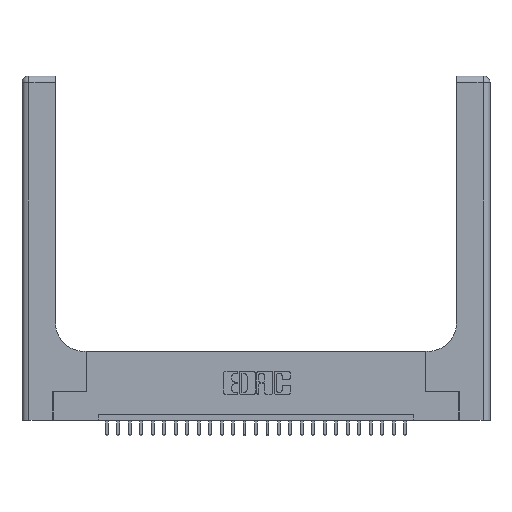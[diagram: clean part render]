
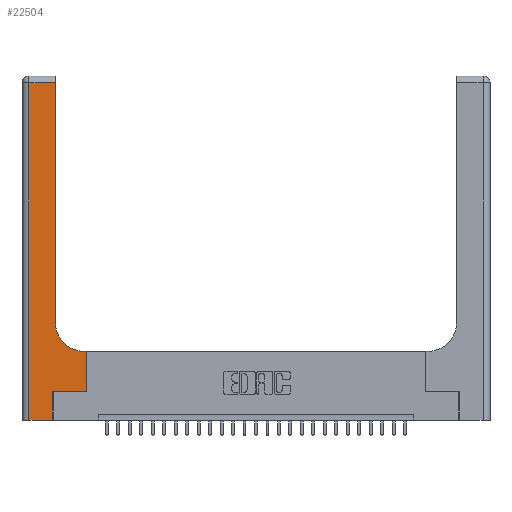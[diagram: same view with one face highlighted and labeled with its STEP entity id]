
A CAD part, top view. The second image highlights one B-rep face of the part: STEP entity #22504.
In plain terms, the highlighted planar face has unit normal (0, 0, 1).
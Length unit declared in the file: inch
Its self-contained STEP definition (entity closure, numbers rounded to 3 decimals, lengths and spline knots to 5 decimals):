
#38 = VECTOR ( 'NONE', #24473, 39.37008 ) ;
#430 = DIRECTION ( 'NONE',  ( -1., 0., 0. ) ) ;
#1986 = LINE ( 'NONE', #11225, #23203 ) ;
#2425 = CIRCLE ( 'NONE', #13487, 0.25 ) ;
#2808 = EDGE_CURVE ( 'NONE', #12086, #2847, #2425, .T. ) ;
#2847 = VERTEX_POINT ( 'NONE', #17193 ) ;
#3329 = VECTOR ( 'NONE', #17822, 39.37008 ) ;
#3611 = VERTEX_POINT ( 'NONE', #10366 ) ;
#3762 = ORIENTED_EDGE ( 'NONE', *, *, #16339, .T. ) ;
#4266 = ORIENTED_EDGE ( 'NONE', *, *, #25864, .T. ) ;
#4330 = CARTESIAN_POINT ( 'NONE',  ( 0.269, 0., 0.37 ) ) ;
#4555 = LINE ( 'NONE', #6784, #12500 ) ;
#5324 = CARTESIAN_POINT ( 'NONE',  ( 0.5585, 0.25, 0.37 ) ) ;
#5474 = CARTESIAN_POINT ( 'NONE',  ( 0., 0., 0.37 ) ) ;
#5897 = ORIENTED_EDGE ( 'NONE', *, *, #21967, .T. ) ;
#6282 = DIRECTION ( 'NONE',  ( 1., 0., 0. ) ) ;
#6784 = CARTESIAN_POINT ( 'NONE',  ( 0.2915, 3., 0.37 ) ) ;
#9397 = ORIENTED_EDGE ( 'NONE', *, *, #18760, .T. ) ;
#9572 = EDGE_LOOP ( 'NONE', ( #24505, #5897, #26247, #18414, #4266, #3762, #9597, #9397, #11626 ) ) ;
#9597 = ORIENTED_EDGE ( 'NONE', *, *, #9991, .T. ) ;
#9695 = CARTESIAN_POINT ( 'NONE',  ( 0.06, 3., 0.37 ) ) ;
#9987 = LINE ( 'NONE', #9695, #14293 ) ;
#9991 = EDGE_CURVE ( 'NONE', #10558, #22808, #16920, .T. ) ;
#10335 = DIRECTION ( 'NONE',  ( 0., 0., -1. ) ) ;
#10366 = CARTESIAN_POINT ( 'NONE',  ( 0.269, 0., 0.37 ) ) ;
#10558 = VERTEX_POINT ( 'NONE', #19305 ) ;
#11225 = CARTESIAN_POINT ( 'NONE',  ( 0.269, 0.25, 0.37 ) ) ;
#11626 = ORIENTED_EDGE ( 'NONE', *, *, #2808, .T. ) ;
#11839 = DIRECTION ( 'NONE',  ( 0., -1., 0. ) ) ;
#11867 = EDGE_CURVE ( 'NONE', #2847, #13558, #4555, .T. ) ;
#12086 = VERTEX_POINT ( 'NONE', #17503 ) ;
#12358 = CARTESIAN_POINT ( 'NONE',  ( 0.2915, 2.94, 0.37 ) ) ;
#12500 = VECTOR ( 'NONE', #23912, 39.37008 ) ;
#12856 = EDGE_CURVE ( 'NONE', #14881, #3611, #15755, .T. ) ;
#13241 = AXIS2_PLACEMENT_3D ( 'NONE', #19711, #21966, #430 ) ;
#13255 = CARTESIAN_POINT ( 'NONE',  ( 0.5585, 0.6, 0.37 ) ) ;
#13269 = DIRECTION ( 'NONE',  ( 1., 0., 0. ) ) ;
#13487 = AXIS2_PLACEMENT_3D ( 'NONE', #14774, #10335, #6282 ) ;
#13558 = VERTEX_POINT ( 'NONE', #12358 ) ;
#14292 = LINE ( 'NONE', #4330, #15610 ) ;
#14293 = VECTOR ( 'NONE', #11839, 39.37008 ) ;
#14421 = CARTESIAN_POINT ( 'NONE',  ( 0.06, 0., 0.37 ) ) ;
#14774 = CARTESIAN_POINT ( 'NONE',  ( 0.5415, 0.85, 0.37 ) ) ;
#14881 = VERTEX_POINT ( 'NONE', #14421 ) ;
#15497 = PLANE ( 'NONE',  #13241 ) ;
#15610 = VECTOR ( 'NONE', #25710, 39.37008 ) ;
#15755 = LINE ( 'NONE', #5474, #17760 ) ;
#15894 = EDGE_CURVE ( 'NONE', #16271, #14881, #9987, .T. ) ;
#15913 = CARTESIAN_POINT ( 'NONE',  ( 0., 2.94, 0.37 ) ) ;
#16271 = VERTEX_POINT ( 'NONE', #24321 ) ;
#16339 = EDGE_CURVE ( 'NONE', #25624, #10558, #1986, .T. ) ;
#16920 = LINE ( 'NONE', #5324, #38 ) ;
#17193 = CARTESIAN_POINT ( 'NONE',  ( 0.2915, 0.85, 0.37 ) ) ;
#17503 = CARTESIAN_POINT ( 'NONE',  ( 0.5415, 0.6, 0.37 ) ) ;
#17760 = VECTOR ( 'NONE', #20239, 39.37008 ) ;
#17822 = DIRECTION ( 'NONE',  ( -1., 0., 0. ) ) ;
#18414 = ORIENTED_EDGE ( 'NONE', *, *, #12856, .T. ) ;
#18652 = CARTESIAN_POINT ( 'NONE',  ( 0.269, 0.25, 0.37 ) ) ;
#18760 = EDGE_CURVE ( 'NONE', #22808, #12086, #26256, .T. ) ;
#19305 = CARTESIAN_POINT ( 'NONE',  ( 0.5585, 0.25, 0.37 ) ) ;
#19692 = CARTESIAN_POINT ( 'NONE',  ( 0.2915, 0.6, 0.37 ) ) ;
#19711 = CARTESIAN_POINT ( 'NONE',  ( 0., 3., 0.37 ) ) ;
#20239 = DIRECTION ( 'NONE',  ( 1., 0., 0. ) ) ;
#21083 = LINE ( 'NONE', #15913, #22074 ) ;
#21966 = DIRECTION ( 'NONE',  ( 0., 0., -1. ) ) ;
#21967 = EDGE_CURVE ( 'NONE', #13558, #16271, #21083, .T. ) ;
#22074 = VECTOR ( 'NONE', #22180, 39.37008 ) ;
#22180 = DIRECTION ( 'NONE',  ( -1., 0., 0. ) ) ;
#22504 = ADVANCED_FACE ( 'NONE', ( #25734 ), #15497, .F. ) ;
#22808 = VERTEX_POINT ( 'NONE', #13255 ) ;
#23203 = VECTOR ( 'NONE', #13269, 39.37008 ) ;
#23912 = DIRECTION ( 'NONE',  ( 0., 1., 0. ) ) ;
#24321 = CARTESIAN_POINT ( 'NONE',  ( 0.06, 2.94, 0.37 ) ) ;
#24473 = DIRECTION ( 'NONE',  ( 0., 1., 0. ) ) ;
#24505 = ORIENTED_EDGE ( 'NONE', *, *, #11867, .T. ) ;
#25624 = VERTEX_POINT ( 'NONE', #18652 ) ;
#25710 = DIRECTION ( 'NONE',  ( 0., 1., 0. ) ) ;
#25734 = FACE_OUTER_BOUND ( 'NONE', #9572, .T. ) ;
#25864 = EDGE_CURVE ( 'NONE', #3611, #25624, #14292, .T. ) ;
#26247 = ORIENTED_EDGE ( 'NONE', *, *, #15894, .T. ) ;
#26256 = LINE ( 'NONE', #19692, #3329 ) ;
